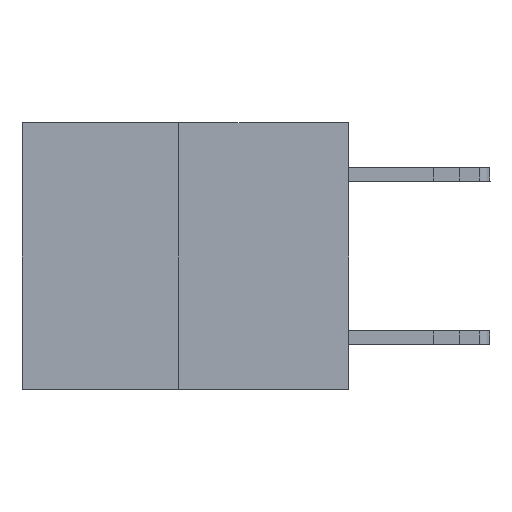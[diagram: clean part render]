
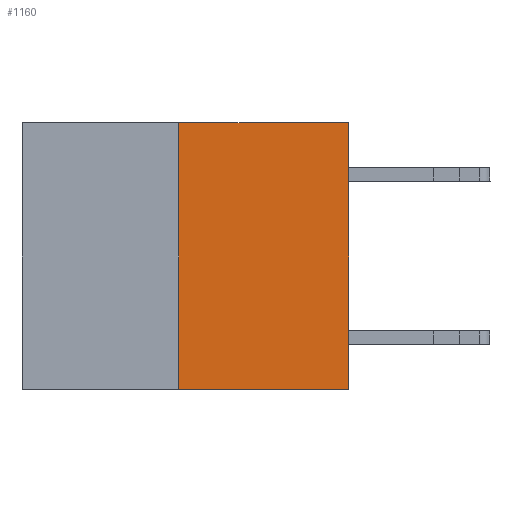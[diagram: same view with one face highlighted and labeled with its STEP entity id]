
A CAD part, left-side view. The second image highlights one B-rep face of the part: STEP entity #1160.
In plain terms, the highlighted planar face has unit normal (-1, 0, 0).
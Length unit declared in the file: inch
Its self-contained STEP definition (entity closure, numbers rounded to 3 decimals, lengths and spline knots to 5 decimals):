
#911 = DIRECTION ( 'NONE',  ( 0., 0., -1. ) ) ;
#1160 = ADVANCED_FACE ( 'NONE', ( #19421 ), #4394, .F. ) ;
#1249 = LINE ( 'NONE', #6930, #14910 ) ;
#1627 = CARTESIAN_POINT ( 'NONE',  ( 0., 0.312, -0.49 ) ) ;
#1910 = AXIS2_PLACEMENT_3D ( 'NONE', #4484, #13260, #911 ) ;
#3483 = VERTEX_POINT ( 'NONE', #1627 ) ;
#4394 = PLANE ( 'NONE',  #1910 ) ;
#4484 = CARTESIAN_POINT ( 'NONE',  ( 0., 0.6, 0. ) ) ;
#5201 = CARTESIAN_POINT ( 'NONE',  ( 0., 0., 0. ) ) ;
#5433 = DIRECTION ( 'NONE',  ( 0., -1., 0. ) ) ;
#6265 = VERTEX_POINT ( 'NONE', #10798 ) ;
#6930 = CARTESIAN_POINT ( 'NONE',  ( 0., 0.6, -0.49 ) ) ;
#7215 = CARTESIAN_POINT ( 'NONE',  ( 0., 0.312, 0. ) ) ;
#9102 = LINE ( 'NONE', #5201, #19380 ) ;
#9997 = ORIENTED_EDGE ( 'NONE', *, *, #17981, .T. ) ;
#10459 = VECTOR ( 'NONE', #13047, 39.37008 ) ;
#10798 = CARTESIAN_POINT ( 'NONE',  ( 0., 0., -0.49 ) ) ;
#11628 = VERTEX_POINT ( 'NONE', #17698 ) ;
#13047 = DIRECTION ( 'NONE',  ( 0., 0., 1. ) ) ;
#13260 = DIRECTION ( 'NONE',  ( 1., 0., 0. ) ) ;
#13736 = EDGE_LOOP ( 'NONE', ( #19314, #9997, #19400, #14178 ) ) ;
#14178 = ORIENTED_EDGE ( 'NONE', *, *, #23816, .F. ) ;
#14901 = CARTESIAN_POINT ( 'NONE',  ( 0., 0.6, 0. ) ) ;
#14910 = VECTOR ( 'NONE', #24831, 39.37008 ) ;
#15038 = CARTESIAN_POINT ( 'NONE',  ( 0., 0.312, -0.49 ) ) ;
#15769 = LINE ( 'NONE', #15038, #10459 ) ;
#15964 = EDGE_CURVE ( 'NONE', #6265, #11628, #9102, .T. ) ;
#16117 = LINE ( 'NONE', #14901, #24737 ) ;
#17698 = CARTESIAN_POINT ( 'NONE',  ( 0., 0., 0. ) ) ;
#17981 = EDGE_CURVE ( 'NONE', #3483, #6265, #1249, .T. ) ;
#19314 = ORIENTED_EDGE ( 'NONE', *, *, #19336, .F. ) ;
#19336 = EDGE_CURVE ( 'NONE', #3483, #24052, #15769, .T. ) ;
#19380 = VECTOR ( 'NONE', #20901, 39.37008 ) ;
#19400 = ORIENTED_EDGE ( 'NONE', *, *, #15964, .T. ) ;
#19421 = FACE_OUTER_BOUND ( 'NONE', #13736, .T. ) ;
#20901 = DIRECTION ( 'NONE',  ( 0., 0., 1. ) ) ;
#23816 = EDGE_CURVE ( 'NONE', #24052, #11628, #16117, .T. ) ;
#24052 = VERTEX_POINT ( 'NONE', #7215 ) ;
#24737 = VECTOR ( 'NONE', #5433, 39.37008 ) ;
#24831 = DIRECTION ( 'NONE',  ( 0., -1., 0. ) ) ;
